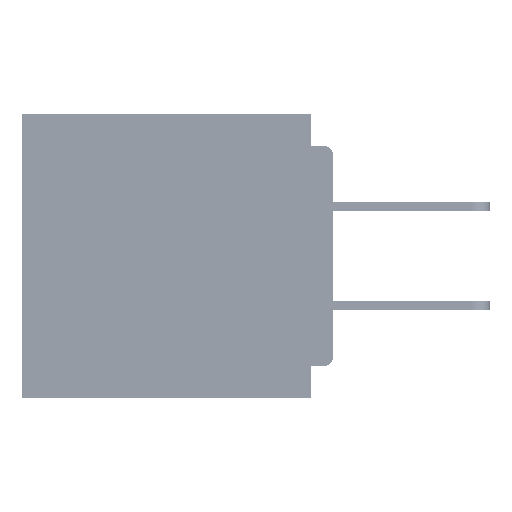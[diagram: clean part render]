
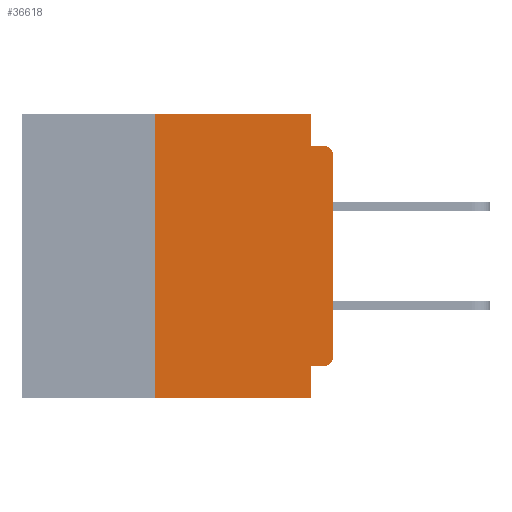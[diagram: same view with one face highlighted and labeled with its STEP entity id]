
A CAD part, left-side view. The second image highlights one B-rep face of the part: STEP entity #36618.
In plain terms, the highlighted planar face has unit normal (-1, 0, 0).
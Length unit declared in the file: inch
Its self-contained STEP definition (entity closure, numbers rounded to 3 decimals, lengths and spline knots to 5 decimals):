
#35 = DIRECTION ( 'NONE',  ( 0., 1., 0. ) ) ;
#284 = VERTEX_POINT ( 'NONE', #39898 ) ;
#716 = ORIENTED_EDGE ( 'NONE', *, *, #25350, .F. ) ;
#2308 = CARTESIAN_POINT ( 'NONE',  ( 0., 0.437, -0.4 ) ) ;
#2771 = LINE ( 'NONE', #59342, #55170 ) ;
#3008 = EDGE_CURVE ( 'NONE', #45492, #53743, #9095, .T. ) ;
#4734 = CARTESIAN_POINT ( 'NONE',  ( 0., 0., -0.355 ) ) ;
#5146 = AXIS2_PLACEMENT_3D ( 'NONE', #9553, #44036, #14533 ) ;
#6570 = VECTOR ( 'NONE', #59993, 39.37008 ) ;
#6574 = CARTESIAN_POINT ( 'NONE',  ( 0., 0., 0. ) ) ;
#6955 = VECTOR ( 'NONE', #26592, 39.37008 ) ;
#7865 = LINE ( 'NONE', #2308, #45677 ) ;
#9095 = LINE ( 'NONE', #6574, #48426 ) ;
#9535 = CIRCLE ( 'NONE', #39496, 0.015 ) ;
#9553 = CARTESIAN_POINT ( 'NONE',  ( 0., 0.437, 0. ) ) ;
#9559 = VERTEX_POINT ( 'NONE', #50142 ) ;
#9574 = CARTESIAN_POINT ( 'NONE',  ( 0., 0.25, -0.4 ) ) ;
#9980 = ORIENTED_EDGE ( 'NONE', *, *, #24448, .F. ) ;
#10229 = CARTESIAN_POINT ( 'NONE',  ( 0., 0.015, -0.34 ) ) ;
#11091 = LINE ( 'NONE', #20350, #48886 ) ;
#13167 = FACE_OUTER_BOUND ( 'NONE', #28289, .T. ) ;
#13520 = EDGE_CURVE ( 'NONE', #61061, #284, #20131, .T. ) ;
#14533 = DIRECTION ( 'NONE',  ( 0., 0., -1. ) ) ;
#15213 = DIRECTION ( 'NONE',  ( 0., 0., -1. ) ) ;
#16724 = EDGE_CURVE ( 'NONE', #284, #59646, #2771, .T. ) ;
#17341 = CARTESIAN_POINT ( 'NONE',  ( 0., 0.015, -0.06 ) ) ;
#18510 = DIRECTION ( 'NONE',  ( 0., 0., -1. ) ) ;
#19063 = EDGE_CURVE ( 'NONE', #22204, #54125, #48365, .T. ) ;
#20131 = LINE ( 'NONE', #46166, #6955 ) ;
#20350 = CARTESIAN_POINT ( 'NONE',  ( 0., 0.25, -0.4 ) ) ;
#21014 = EDGE_CURVE ( 'NONE', #22204, #45492, #9535, .T. ) ;
#21773 = DIRECTION ( 'NONE',  ( 0., -1., 0. ) ) ;
#22193 = VECTOR ( 'NONE', #35, 39.37008 ) ;
#22204 = VERTEX_POINT ( 'NONE', #63783 ) ;
#22329 = DIRECTION ( 'NONE',  ( 0., 0., -1. ) ) ;
#24448 = EDGE_CURVE ( 'NONE', #54125, #30383, #32991, .T. ) ;
#25350 = EDGE_CURVE ( 'NONE', #59646, #9559, #31304, .T. ) ;
#26592 = DIRECTION ( 'NONE',  ( 0., -1., 0. ) ) ;
#28289 = EDGE_LOOP ( 'NONE', ( #43725, #55956, #716, #36763, #62958, #34856, #45428, #9980, #58996, #44181 ) ) ;
#29866 = DIRECTION ( 'NONE',  ( 0., 0., -1. ) ) ;
#30383 = VERTEX_POINT ( 'NONE', #43726 ) ;
#31304 = LINE ( 'NONE', #45108, #6570 ) ;
#32991 = LINE ( 'NONE', #48012, #59158 ) ;
#33982 = CARTESIAN_POINT ( 'NONE',  ( 0., 0., -0.34 ) ) ;
#34187 = PLANE ( 'NONE',  #5146 ) ;
#34639 = CARTESIAN_POINT ( 'NONE',  ( 0., 0.031, -0.045 ) ) ;
#34856 = ORIENTED_EDGE ( 'NONE', *, *, #60245, .F. ) ;
#36618 = ADVANCED_FACE ( 'NONE', ( #13167 ), #34187, .F. ) ;
#36763 = ORIENTED_EDGE ( 'NONE', *, *, #16724, .F. ) ;
#39496 = AXIS2_PLACEMENT_3D ( 'NONE', #10229, #44734, #15213 ) ;
#39898 = CARTESIAN_POINT ( 'NONE',  ( 0., 0.031, 0. ) ) ;
#41071 = DIRECTION ( 'NONE',  ( 0., 0., 1. ) ) ;
#43725 = ORIENTED_EDGE ( 'NONE', *, *, #3008, .T. ) ;
#43726 = CARTESIAN_POINT ( 'NONE',  ( 0., 0.031, -0.4 ) ) ;
#44036 = DIRECTION ( 'NONE',  ( 1., 0., 0. ) ) ;
#44181 = ORIENTED_EDGE ( 'NONE', *, *, #21014, .T. ) ;
#44734 = DIRECTION ( 'NONE',  ( -1., 0., 0. ) ) ;
#45108 = CARTESIAN_POINT ( 'NONE',  ( 0., 0., -0.045 ) ) ;
#45428 = ORIENTED_EDGE ( 'NONE', *, *, #55791, .T. ) ;
#45492 = VERTEX_POINT ( 'NONE', #33982 ) ;
#45677 = VECTOR ( 'NONE', #21773, 39.37008 ) ;
#46166 = CARTESIAN_POINT ( 'NONE',  ( 0., 0.437, 0. ) ) ;
#48012 = CARTESIAN_POINT ( 'NONE',  ( 0., 0.031, -0.4 ) ) ;
#48365 = LINE ( 'NONE', #4734, #22193 ) ;
#48426 = VECTOR ( 'NONE', #41071, 39.37008 ) ;
#48886 = VECTOR ( 'NONE', #54745, 39.37008 ) ;
#50142 = CARTESIAN_POINT ( 'NONE',  ( 0., 0.015, -0.045 ) ) ;
#51783 = DIRECTION ( 'NONE',  ( -1., 0., 0. ) ) ;
#53505 = CIRCLE ( 'NONE', #59386, 0.015 ) ;
#53743 = VERTEX_POINT ( 'NONE', #56580 ) ;
#54125 = VERTEX_POINT ( 'NONE', #59407 ) ;
#54399 = EDGE_CURVE ( 'NONE', #53743, #9559, #53505, .T. ) ;
#54745 = DIRECTION ( 'NONE',  ( 0., 0., 1. ) ) ;
#55170 = VECTOR ( 'NONE', #29866, 39.37008 ) ;
#55791 = EDGE_CURVE ( 'NONE', #63441, #30383, #7865, .T. ) ;
#55956 = ORIENTED_EDGE ( 'NONE', *, *, #54399, .T. ) ;
#56580 = CARTESIAN_POINT ( 'NONE',  ( 0., 0., -0.06 ) ) ;
#58996 = ORIENTED_EDGE ( 'NONE', *, *, #19063, .F. ) ;
#59158 = VECTOR ( 'NONE', #18510, 39.37008 ) ;
#59342 = CARTESIAN_POINT ( 'NONE',  ( 0., 0.031, 0. ) ) ;
#59386 = AXIS2_PLACEMENT_3D ( 'NONE', #17341, #51783, #22329 ) ;
#59407 = CARTESIAN_POINT ( 'NONE',  ( 0., 0.031, -0.355 ) ) ;
#59646 = VERTEX_POINT ( 'NONE', #34639 ) ;
#59993 = DIRECTION ( 'NONE',  ( 0., -1., 0. ) ) ;
#60245 = EDGE_CURVE ( 'NONE', #63441, #61061, #11091, .T. ) ;
#60948 = CARTESIAN_POINT ( 'NONE',  ( 0., 0.25, 0. ) ) ;
#61061 = VERTEX_POINT ( 'NONE', #60948 ) ;
#62958 = ORIENTED_EDGE ( 'NONE', *, *, #13520, .F. ) ;
#63441 = VERTEX_POINT ( 'NONE', #9574 ) ;
#63783 = CARTESIAN_POINT ( 'NONE',  ( 0., 0.015, -0.355 ) ) ;
